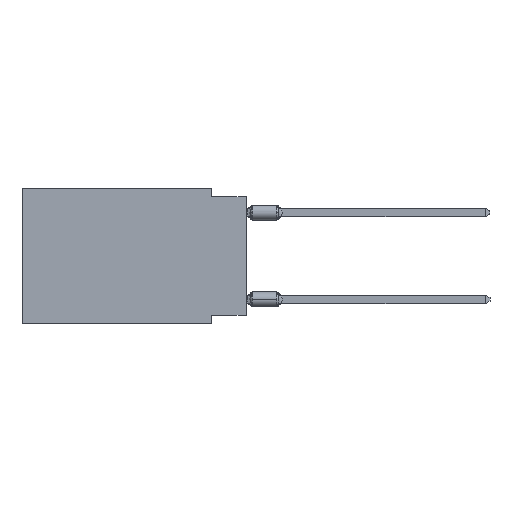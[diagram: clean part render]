
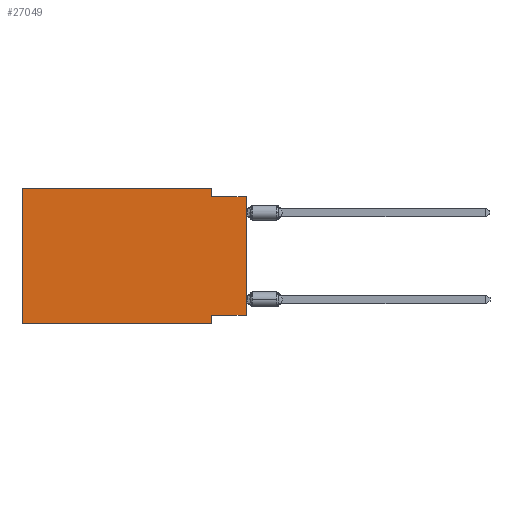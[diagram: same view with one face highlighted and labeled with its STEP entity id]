
A CAD part, left-side view. The second image highlights one B-rep face of the part: STEP entity #27049.
In plain terms, the highlighted planar face has unit normal (-1, 0, 0).
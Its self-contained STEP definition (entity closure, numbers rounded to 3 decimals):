
#412 = EDGE_CURVE ( 'NONE', #17421, #29705, #16157, .T. ) ;
#451 = DIRECTION ( 'NONE',  ( 0., -1., 0. ) ) ;
#1056 = CARTESIAN_POINT ( 'NONE',  ( 0., 16.383, 0. ) ) ;
#1314 = CARTESIAN_POINT ( 'NONE',  ( 0., 0., -9.271 ) ) ;
#1652 = LINE ( 'NONE', #16837, #11880 ) ;
#1715 = CARTESIAN_POINT ( 'NONE',  ( 0., 0., -9.271 ) ) ;
#1792 = ORIENTED_EDGE ( 'NONE', *, *, #4258, .T. ) ;
#1838 = DIRECTION ( 'NONE',  ( 0., -1., 0. ) ) ;
#2204 = LINE ( 'NONE', #4529, #20835 ) ;
#2506 = CARTESIAN_POINT ( 'NONE',  ( 0., 16.383, -9.906 ) ) ;
#2918 = ORIENTED_EDGE ( 'NONE', *, *, #412, .F. ) ;
#3221 = ORIENTED_EDGE ( 'NONE', *, *, #30194, .F. ) ;
#4258 = EDGE_CURVE ( 'NONE', #17421, #10586, #18288, .T. ) ;
#4529 = CARTESIAN_POINT ( 'NONE',  ( 0., 2.54, 0. ) ) ;
#4590 = VECTOR ( 'NONE', #26345, 1000. ) ;
#4709 = EDGE_CURVE ( 'NONE', #19621, #26117, #12964, .T. ) ;
#6093 = LINE ( 'NONE', #10553, #11300 ) ;
#6489 = DIRECTION ( 'NONE',  ( 0., 0., -1. ) ) ;
#8653 = EDGE_CURVE ( 'NONE', #19100, #19621, #18938, .T. ) ;
#8732 = DIRECTION ( 'NONE',  ( 0., 0., -1. ) ) ;
#8988 = ORIENTED_EDGE ( 'NONE', *, *, #4709, .F. ) ;
#9042 = DIRECTION ( 'NONE',  ( 0., 0., 1. ) ) ;
#9174 = CARTESIAN_POINT ( 'NONE',  ( 0., 2.54, -9.271 ) ) ;
#10553 = CARTESIAN_POINT ( 'NONE',  ( 0., 2.54, -9.906 ) ) ;
#10586 = VERTEX_POINT ( 'NONE', #22978 ) ;
#11156 = EDGE_CURVE ( 'NONE', #27004, #10586, #31677, .T. ) ;
#11300 = VECTOR ( 'NONE', #8732, 1000. ) ;
#11880 = VECTOR ( 'NONE', #29180, 1000. ) ;
#12770 = VECTOR ( 'NONE', #9042, 1000. ) ;
#12964 = LINE ( 'NONE', #23003, #30324 ) ;
#14091 = VERTEX_POINT ( 'NONE', #17734 ) ;
#14582 = DIRECTION ( 'NONE',  ( 0., 0., -1. ) ) ;
#15962 = CARTESIAN_POINT ( 'NONE',  ( 0., 2.54, 0. ) ) ;
#16157 = LINE ( 'NONE', #1314, #4590 ) ;
#16837 = CARTESIAN_POINT ( 'NONE',  ( 0., 16.383, -9.906 ) ) ;
#17421 = VERTEX_POINT ( 'NONE', #1715 ) ;
#17734 = CARTESIAN_POINT ( 'NONE',  ( 0., 2.54, -9.906 ) ) ;
#17952 = CARTESIAN_POINT ( 'NONE',  ( 0., 16.383, 0. ) ) ;
#18288 = LINE ( 'NONE', #25685, #21856 ) ;
#18938 = LINE ( 'NONE', #28987, #12770 ) ;
#19100 = VERTEX_POINT ( 'NONE', #2506 ) ;
#19527 = ORIENTED_EDGE ( 'NONE', *, *, #8653, .F. ) ;
#19621 = VERTEX_POINT ( 'NONE', #17952 ) ;
#20835 = VECTOR ( 'NONE', #14582, 1000. ) ;
#21147 = DIRECTION ( 'NONE',  ( 1., 0., 0. ) ) ;
#21483 = FACE_OUTER_BOUND ( 'NONE', #25861, .T. ) ;
#21615 = EDGE_CURVE ( 'NONE', #19100, #14091, #1652, .T. ) ;
#21856 = VECTOR ( 'NONE', #22714, 1000. ) ;
#22714 = DIRECTION ( 'NONE',  ( 0., 0., 1. ) ) ;
#22978 = CARTESIAN_POINT ( 'NONE',  ( 0., 0., -0.635 ) ) ;
#23003 = CARTESIAN_POINT ( 'NONE',  ( 0., 16.383, 0. ) ) ;
#23628 = CARTESIAN_POINT ( 'NONE',  ( 0., 2.54, -0.635 ) ) ;
#24401 = CARTESIAN_POINT ( 'NONE',  ( 0., 0., -0.635 ) ) ;
#25685 = CARTESIAN_POINT ( 'NONE',  ( 0., 0., 0. ) ) ;
#25861 = EDGE_LOOP ( 'NONE', ( #1792, #32075, #3221, #8988, #19527, #27432, #27182, #2918 ) ) ;
#26117 = VERTEX_POINT ( 'NONE', #15962 ) ;
#26345 = DIRECTION ( 'NONE',  ( 0., 1., 0. ) ) ;
#26959 = VECTOR ( 'NONE', #1838, 1000. ) ;
#27004 = VERTEX_POINT ( 'NONE', #23628 ) ;
#27049 = ADVANCED_FACE ( 'NONE', ( #21483 ), #29062, .F. ) ;
#27182 = ORIENTED_EDGE ( 'NONE', *, *, #30856, .F. ) ;
#27432 = ORIENTED_EDGE ( 'NONE', *, *, #21615, .T. ) ;
#28987 = CARTESIAN_POINT ( 'NONE',  ( 0., 16.383, 0. ) ) ;
#29062 = PLANE ( 'NONE',  #31060 ) ;
#29180 = DIRECTION ( 'NONE',  ( 0., -1., 0. ) ) ;
#29705 = VERTEX_POINT ( 'NONE', #9174 ) ;
#30194 = EDGE_CURVE ( 'NONE', #26117, #27004, #2204, .T. ) ;
#30324 = VECTOR ( 'NONE', #451, 1000. ) ;
#30856 = EDGE_CURVE ( 'NONE', #29705, #14091, #6093, .T. ) ;
#31060 = AXIS2_PLACEMENT_3D ( 'NONE', #1056, #21147, #6489 ) ;
#31677 = LINE ( 'NONE', #24401, #26959 ) ;
#32075 = ORIENTED_EDGE ( 'NONE', *, *, #11156, .F. ) ;
